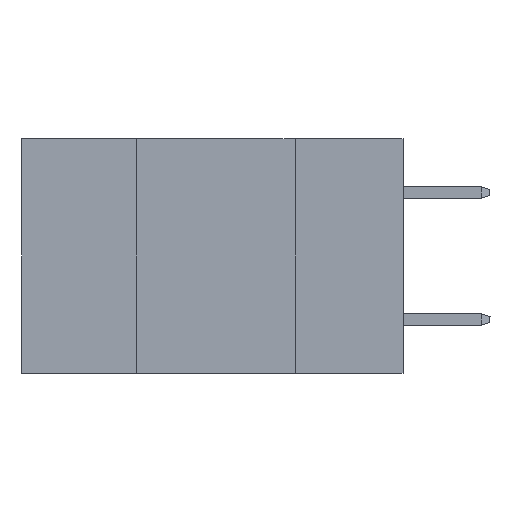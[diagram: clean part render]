
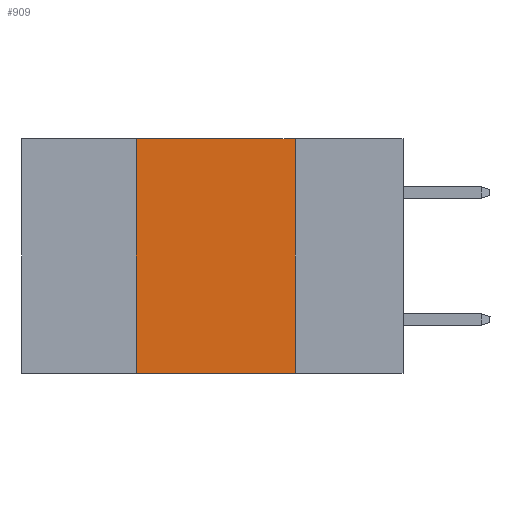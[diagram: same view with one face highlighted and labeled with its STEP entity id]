
A CAD part, left-side view. The second image highlights one B-rep face of the part: STEP entity #909.
In plain terms, the highlighted planar face has unit normal (-1, 0, 0).
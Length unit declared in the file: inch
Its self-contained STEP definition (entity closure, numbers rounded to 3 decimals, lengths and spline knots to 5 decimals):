
#909 = ADVANCED_FACE ( 'NONE', ( #2613 ), #9837, .F. ) ;
#973 = CARTESIAN_POINT ( 'NONE',  ( 0., 0.6, 0. ) ) ;
#2469 = CARTESIAN_POINT ( 'NONE',  ( 0., 0.6, 0. ) ) ;
#2613 = FACE_OUTER_BOUND ( 'NONE', #12629, .T. ) ;
#4155 = VERTEX_POINT ( 'NONE', #15260 ) ;
#4648 = ORIENTED_EDGE ( 'NONE', *, *, #12350, .F. ) ;
#4737 = VECTOR ( 'NONE', #23049, 39.37008 ) ;
#5357 = EDGE_CURVE ( 'NONE', #10330, #18668, #20102, .T. ) ;
#5450 = VECTOR ( 'NONE', #22233, 39.37008 ) ;
#5743 = VECTOR ( 'NONE', #9563, 39.37008 ) ;
#5986 = CARTESIAN_POINT ( 'NONE',  ( 0., 0.17, 0. ) ) ;
#6480 = LINE ( 'NONE', #10325, #4737 ) ;
#8612 = VERTEX_POINT ( 'NONE', #21916 ) ;
#8786 = EDGE_CURVE ( 'NONE', #8612, #18668, #6480, .T. ) ;
#9563 = DIRECTION ( 'NONE',  ( 0., 0., -1. ) ) ;
#9837 = PLANE ( 'NONE',  #14376 ) ;
#10325 = CARTESIAN_POINT ( 'NONE',  ( 0., 0.6, -0.37 ) ) ;
#10330 = VERTEX_POINT ( 'NONE', #11623 ) ;
#11623 = CARTESIAN_POINT ( 'NONE',  ( 0., 0.17, 0. ) ) ;
#12066 = EDGE_CURVE ( 'NONE', #8612, #4155, #15544, .T. ) ;
#12350 = EDGE_CURVE ( 'NONE', #4155, #10330, #17047, .T. ) ;
#12629 = EDGE_LOOP ( 'NONE', ( #18924, #4648, #14066, #17997 ) ) ;
#14066 = ORIENTED_EDGE ( 'NONE', *, *, #12066, .F. ) ;
#14376 = AXIS2_PLACEMENT_3D ( 'NONE', #973, #15303, #16864 ) ;
#15063 = CARTESIAN_POINT ( 'NONE',  ( 0., 0.42, 0. ) ) ;
#15260 = CARTESIAN_POINT ( 'NONE',  ( 0., 0.42, 0. ) ) ;
#15303 = DIRECTION ( 'NONE',  ( 1., 0., 0. ) ) ;
#15544 = LINE ( 'NONE', #15063, #5450 ) ;
#16864 = DIRECTION ( 'NONE',  ( 0., 0., -1. ) ) ;
#17047 = LINE ( 'NONE', #2469, #18375 ) ;
#17997 = ORIENTED_EDGE ( 'NONE', *, *, #8786, .T. ) ;
#18375 = VECTOR ( 'NONE', #20465, 39.37008 ) ;
#18668 = VERTEX_POINT ( 'NONE', #19954 ) ;
#18924 = ORIENTED_EDGE ( 'NONE', *, *, #5357, .F. ) ;
#19954 = CARTESIAN_POINT ( 'NONE',  ( 0., 0.17, -0.37 ) ) ;
#20102 = LINE ( 'NONE', #5986, #5743 ) ;
#20465 = DIRECTION ( 'NONE',  ( 0., -1., 0. ) ) ;
#21916 = CARTESIAN_POINT ( 'NONE',  ( 0., 0.42, -0.37 ) ) ;
#22233 = DIRECTION ( 'NONE',  ( 0., 0., 1. ) ) ;
#23049 = DIRECTION ( 'NONE',  ( 0., -1., 0. ) ) ;
